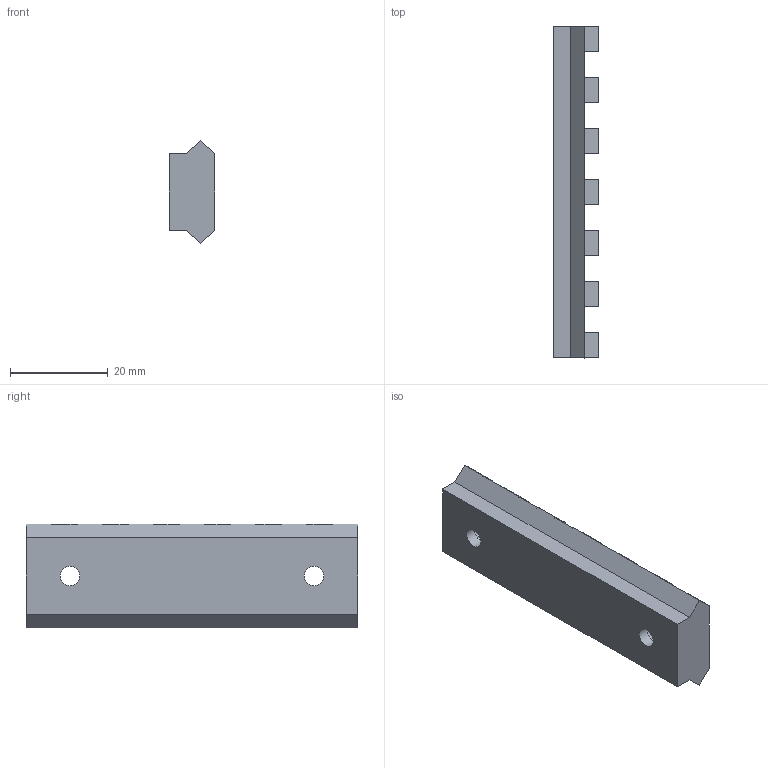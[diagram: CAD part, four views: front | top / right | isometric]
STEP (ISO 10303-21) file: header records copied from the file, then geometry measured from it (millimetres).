
FILE_DESCRIPTION(/* description */ (''),/* implementation_level */ '2;1');
FILE_NAME(/* name */ 'Picatinny Rails v2.step',/* time_stamp */ '2020-06-28T23:20:43-04:00',/* author */ (''),/* organization */ (''),/* preprocessor_version */ 'ST-DEVELOPER v18.1',/* originating_system */ 'Autodesk Translation Framework v9.3.0.1241',/* authorisation */ '');
FILE_SCHEMA (('AUTOMOTIVE_DESIGN { 1 0 10303 214 3 1 1 }'));
Length unit declared in the file: millimetre
Products named in the file (2): Picatinny Rails; Rail
Assembly tree (1 placements, depth 2):
  Picatinny Rails
    Rail
Bounding box: 9.32 x 68.02 x 21.21 mm (x, y, z)
Volume: 8894.1 mm3; surface area: 4794.3 mm2
Topology: 1 solids, 1 shells, 54 faces, 144 edges, 92 vertices
Faces by surface type: plane 50, cylinder 4
Full cylindrical faces by diameter (mm): 4 x2, 7 x1, 7.25 x1
Entity records: 1701 total; most frequent: CARTESIAN_POINT 293, ORIENTED_EDGE 288, DIRECTION 270, EDGE_CURVE 144, LINE 132, VECTOR 132, VERTEX_POINT 92, AXIS2_PLACEMENT_3D 69
